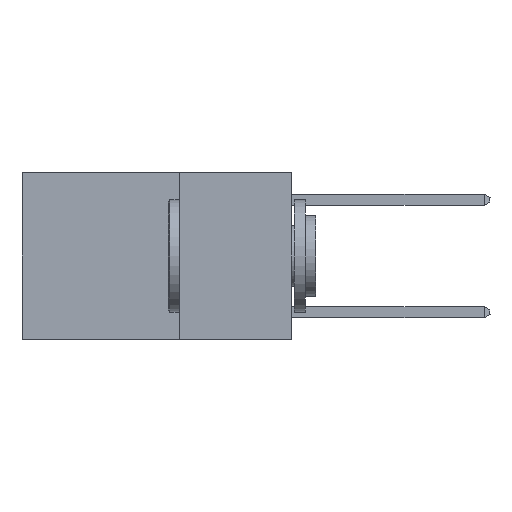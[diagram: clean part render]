
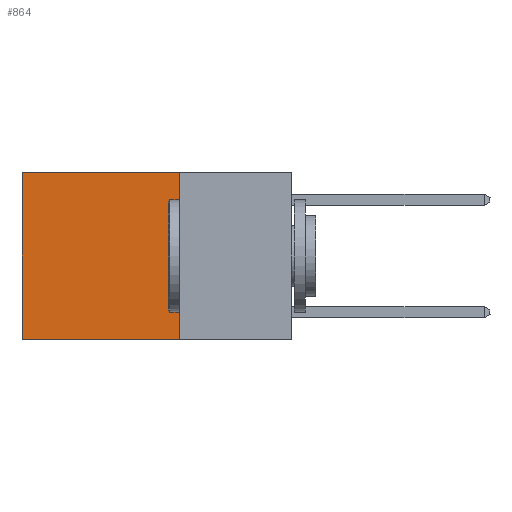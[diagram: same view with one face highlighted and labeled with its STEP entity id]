
A CAD part, left-side view. The second image highlights one B-rep face of the part: STEP entity #864.
In plain terms, the highlighted planar face has unit normal (-1, 0, 0).
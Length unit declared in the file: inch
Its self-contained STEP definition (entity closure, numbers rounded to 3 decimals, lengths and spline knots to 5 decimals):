
#143 = LINE ( 'NONE', #4943, #5999 ) ;
#467 = ORIENTED_EDGE ( 'NONE', *, *, #11494, .T. ) ;
#864 = ADVANCED_FACE ( 'NONE', ( #7642 ), #11226, .F. ) ;
#924 = LINE ( 'NONE', #7608, #2804 ) ;
#1541 = LINE ( 'NONE', #10521, #1544 ) ;
#1544 = VECTOR ( 'NONE', #14055, 39.37008 ) ;
#1612 = VERTEX_POINT ( 'NONE', #10621 ) ;
#1883 = LINE ( 'NONE', #6364, #5617 ) ;
#2796 = EDGE_CURVE ( 'NONE', #9335, #6455, #924, .T. ) ;
#2804 = VECTOR ( 'NONE', #5487, 39.37008 ) ;
#3874 = VERTEX_POINT ( 'NONE', #12760 ) ;
#4619 = ORIENTED_EDGE ( 'NONE', *, *, #2796, .T. ) ;
#4643 = DIRECTION ( 'NONE',  ( 0., 1., 0. ) ) ;
#4943 = CARTESIAN_POINT ( 'NONE',  ( 0.2625, 0.25, -0.37 ) ) ;
#5262 = ORIENTED_EDGE ( 'NONE', *, *, #6250, .F. ) ;
#5487 = DIRECTION ( 'NONE',  ( 0., 1., 0. ) ) ;
#5617 = VECTOR ( 'NONE', #10850, 39.37008 ) ;
#5999 = VECTOR ( 'NONE', #4643, 39.37008 ) ;
#6250 = EDGE_CURVE ( 'NONE', #1612, #3874, #143, .T. ) ;
#6364 = CARTESIAN_POINT ( 'NONE',  ( 0.2625, 0.6, 0. ) ) ;
#6455 = VERTEX_POINT ( 'NONE', #6847 ) ;
#6847 = CARTESIAN_POINT ( 'NONE',  ( 0.2625, 0.6, 0. ) ) ;
#7608 = CARTESIAN_POINT ( 'NONE',  ( 0.2625, 0.25, 0. ) ) ;
#7642 = FACE_OUTER_BOUND ( 'NONE', #9448, .T. ) ;
#7969 = EDGE_CURVE ( 'NONE', #9335, #1612, #1541, .T. ) ;
#8818 = CARTESIAN_POINT ( 'NONE',  ( 0.2625, 0.25, 0. ) ) ;
#8887 = DIRECTION ( 'NONE',  ( 0., 0., -1. ) ) ;
#9335 = VERTEX_POINT ( 'NONE', #14143 ) ;
#9448 = EDGE_LOOP ( 'NONE', ( #467, #5262, #10023, #4619 ) ) ;
#10023 = ORIENTED_EDGE ( 'NONE', *, *, #7969, .F. ) ;
#10486 = AXIS2_PLACEMENT_3D ( 'NONE', #8818, #14465, #8887 ) ;
#10521 = CARTESIAN_POINT ( 'NONE',  ( 0.2625, 0.25, 0. ) ) ;
#10621 = CARTESIAN_POINT ( 'NONE',  ( 0.2625, 0.25, -0.37 ) ) ;
#10850 = DIRECTION ( 'NONE',  ( 0., 0., -1. ) ) ;
#11226 = PLANE ( 'NONE',  #10486 ) ;
#11494 = EDGE_CURVE ( 'NONE', #6455, #3874, #1883, .T. ) ;
#12760 = CARTESIAN_POINT ( 'NONE',  ( 0.2625, 0.6, -0.37 ) ) ;
#14055 = DIRECTION ( 'NONE',  ( 0., 0., -1. ) ) ;
#14143 = CARTESIAN_POINT ( 'NONE',  ( 0.2625, 0.25, 0. ) ) ;
#14465 = DIRECTION ( 'NONE',  ( 1., 0., 0. ) ) ;
